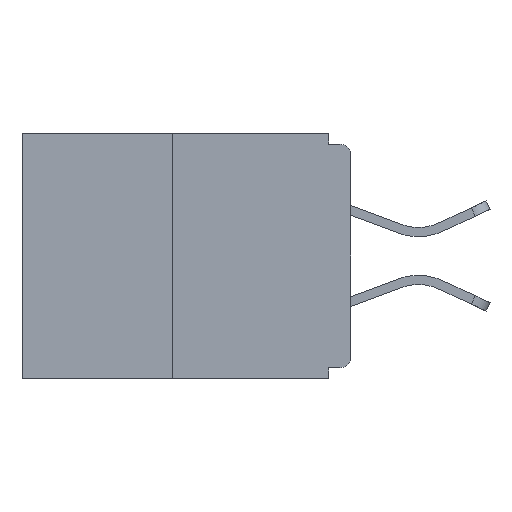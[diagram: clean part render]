
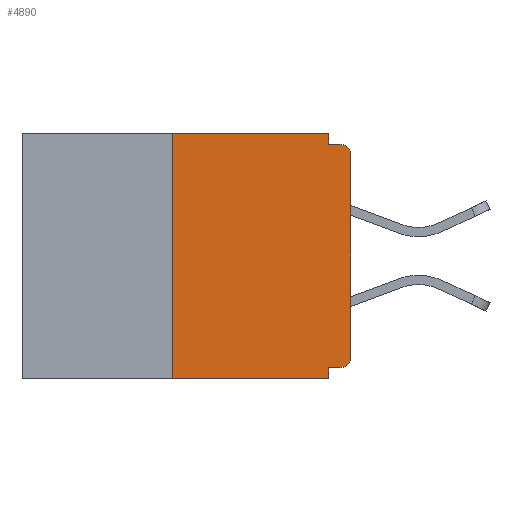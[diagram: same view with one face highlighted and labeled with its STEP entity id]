
A CAD part, left-side view. The second image highlights one B-rep face of the part: STEP entity #4890.
In plain terms, the highlighted planar face has unit normal (-1, 0, 0).
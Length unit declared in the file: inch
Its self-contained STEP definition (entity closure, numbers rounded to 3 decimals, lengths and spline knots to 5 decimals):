
#404 = DIRECTION ( 'NONE',  ( 0., 0., -1. ) ) ;
#408 = CARTESIAN_POINT ( 'NONE',  ( 0., 0.031, -0.343 ) ) ;
#503 = VERTEX_POINT ( 'NONE', #18126 ) ;
#686 = DIRECTION ( 'NONE',  ( 0., -1., 0. ) ) ;
#946 = VERTEX_POINT ( 'NONE', #4311 ) ;
#1173 = CARTESIAN_POINT ( 'NONE',  ( 0., 0.031, -0.328 ) ) ;
#1231 = ORIENTED_EDGE ( 'NONE', *, *, #18230, .T. ) ;
#1665 = DIRECTION ( 'NONE',  ( 0., 0., -1. ) ) ;
#1673 = DIRECTION ( 'NONE',  ( -1., 0., 0. ) ) ;
#1881 = EDGE_CURVE ( 'NONE', #503, #14232, #12226, .T. ) ;
#2849 = CARTESIAN_POINT ( 'NONE',  ( 0., 0.25, -0.343 ) ) ;
#2924 = CIRCLE ( 'NONE', #9737, 0.015 ) ;
#3077 = EDGE_LOOP ( 'NONE', ( #8338, #15510, #16938, #13456, #13620, #15314, #1231, #6418, #14183, #8912 ) ) ;
#3089 = CARTESIAN_POINT ( 'NONE',  ( 0., 0.031, -0.015 ) ) ;
#3169 = VECTOR ( 'NONE', #4947, 39.37008 ) ;
#3208 = EDGE_CURVE ( 'NONE', #9757, #503, #11251, .T. ) ;
#3486 = CARTESIAN_POINT ( 'NONE',  ( 0., 0.015, -0.015 ) ) ;
#3547 = CARTESIAN_POINT ( 'NONE',  ( 0., 0.46, -0.343 ) ) ;
#3639 = DIRECTION ( 'NONE',  ( 0., 1., 0. ) ) ;
#3709 = CARTESIAN_POINT ( 'NONE',  ( 0., 0., 0. ) ) ;
#3763 = CARTESIAN_POINT ( 'NONE',  ( 0., 0., -0.328 ) ) ;
#4077 = VECTOR ( 'NONE', #14711, 39.37008 ) ;
#4293 = VECTOR ( 'NONE', #10420, 39.37008 ) ;
#4311 = CARTESIAN_POINT ( 'NONE',  ( 0., 0., -0.03 ) ) ;
#4638 = CARTESIAN_POINT ( 'NONE',  ( 0., 0.015, -0.03 ) ) ;
#4890 = ADVANCED_FACE ( 'NONE', ( #14898 ), #17347, .F. ) ;
#4947 = DIRECTION ( 'NONE',  ( 0., 0., 1. ) ) ;
#5029 = CARTESIAN_POINT ( 'NONE',  ( 0., 0.015, -0.313 ) ) ;
#6418 = ORIENTED_EDGE ( 'NONE', *, *, #11932, .T. ) ;
#6525 = DIRECTION ( 'NONE',  ( 0., 0., -1. ) ) ;
#6685 = VECTOR ( 'NONE', #404, 39.37008 ) ;
#7086 = CARTESIAN_POINT ( 'NONE',  ( 0., 0.015, -0.328 ) ) ;
#7531 = CIRCLE ( 'NONE', #7698, 0.015 ) ;
#7698 = AXIS2_PLACEMENT_3D ( 'NONE', #4638, #16544, #1665 ) ;
#7897 = CARTESIAN_POINT ( 'NONE',  ( 0., 0.25, 0. ) ) ;
#8244 = VECTOR ( 'NONE', #10811, 39.37008 ) ;
#8338 = ORIENTED_EDGE ( 'NONE', *, *, #3208, .F. ) ;
#8668 = VERTEX_POINT ( 'NONE', #7086 ) ;
#8912 = ORIENTED_EDGE ( 'NONE', *, *, #1881, .F. ) ;
#9363 = CARTESIAN_POINT ( 'NONE',  ( 0., 0., -0.313 ) ) ;
#9737 = AXIS2_PLACEMENT_3D ( 'NONE', #5029, #1673, #6525 ) ;
#9757 = VERTEX_POINT ( 'NONE', #7897 ) ;
#9847 = DIRECTION ( 'NONE',  ( 0., 0., -1. ) ) ;
#10361 = VECTOR ( 'NONE', #3639, 39.37008 ) ;
#10420 = DIRECTION ( 'NONE',  ( 0., 0., -1. ) ) ;
#10547 = LINE ( 'NONE', #3547, #13313 ) ;
#10574 = VECTOR ( 'NONE', #13979, 39.37008 ) ;
#10811 = DIRECTION ( 'NONE',  ( 0., -1., 0. ) ) ;
#11076 = EDGE_CURVE ( 'NONE', #14232, #13512, #13328, .T. ) ;
#11193 = EDGE_CURVE ( 'NONE', #19080, #15170, #10547, .T. ) ;
#11251 = LINE ( 'NONE', #18372, #8244 ) ;
#11261 = LINE ( 'NONE', #3709, #3169 ) ;
#11482 = LINE ( 'NONE', #18004, #4293 ) ;
#11565 = VERTEX_POINT ( 'NONE', #9363 ) ;
#11932 = EDGE_CURVE ( 'NONE', #946, #13512, #7531, .T. ) ;
#12226 = LINE ( 'NONE', #13712, #6685 ) ;
#13007 = AXIS2_PLACEMENT_3D ( 'NONE', #15718, #18740, #9847 ) ;
#13313 = VECTOR ( 'NONE', #686, 39.37008 ) ;
#13328 = LINE ( 'NONE', #16282, #4077 ) ;
#13351 = LINE ( 'NONE', #3763, #10361 ) ;
#13456 = ORIENTED_EDGE ( 'NONE', *, *, #18409, .F. ) ;
#13512 = VERTEX_POINT ( 'NONE', #3486 ) ;
#13620 = ORIENTED_EDGE ( 'NONE', *, *, #17357, .F. ) ;
#13712 = CARTESIAN_POINT ( 'NONE',  ( 0., 0.031, 0. ) ) ;
#13979 = DIRECTION ( 'NONE',  ( 0., 0., 1. ) ) ;
#14183 = ORIENTED_EDGE ( 'NONE', *, *, #11076, .F. ) ;
#14232 = VERTEX_POINT ( 'NONE', #3089 ) ;
#14711 = DIRECTION ( 'NONE',  ( 0., -1., 0. ) ) ;
#14898 = FACE_OUTER_BOUND ( 'NONE', #3077, .T. ) ;
#15170 = VERTEX_POINT ( 'NONE', #408 ) ;
#15314 = ORIENTED_EDGE ( 'NONE', *, *, #18055, .T. ) ;
#15510 = ORIENTED_EDGE ( 'NONE', *, *, #18240, .F. ) ;
#15718 = CARTESIAN_POINT ( 'NONE',  ( 0., 0.46, 0. ) ) ;
#16282 = CARTESIAN_POINT ( 'NONE',  ( 0., 0., -0.015 ) ) ;
#16544 = DIRECTION ( 'NONE',  ( -1., 0., 0. ) ) ;
#16781 = VERTEX_POINT ( 'NONE', #1173 ) ;
#16938 = ORIENTED_EDGE ( 'NONE', *, *, #11193, .T. ) ;
#17347 = PLANE ( 'NONE',  #13007 ) ;
#17357 = EDGE_CURVE ( 'NONE', #8668, #16781, #13351, .T. ) ;
#18004 = CARTESIAN_POINT ( 'NONE',  ( 0., 0.031, -0.343 ) ) ;
#18055 = EDGE_CURVE ( 'NONE', #8668, #11565, #2924, .T. ) ;
#18126 = CARTESIAN_POINT ( 'NONE',  ( 0., 0.031, 0. ) ) ;
#18230 = EDGE_CURVE ( 'NONE', #11565, #946, #11261, .T. ) ;
#18240 = EDGE_CURVE ( 'NONE', #19080, #9757, #18449, .T. ) ;
#18342 = CARTESIAN_POINT ( 'NONE',  ( 0., 0.25, 0. ) ) ;
#18372 = CARTESIAN_POINT ( 'NONE',  ( 0., 0.46, 0. ) ) ;
#18409 = EDGE_CURVE ( 'NONE', #16781, #15170, #11482, .T. ) ;
#18449 = LINE ( 'NONE', #18342, #10574 ) ;
#18740 = DIRECTION ( 'NONE',  ( 1., 0., 0. ) ) ;
#19080 = VERTEX_POINT ( 'NONE', #2849 ) ;
